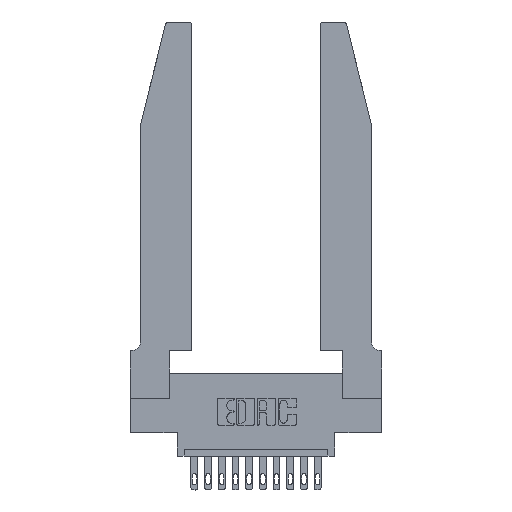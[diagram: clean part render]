
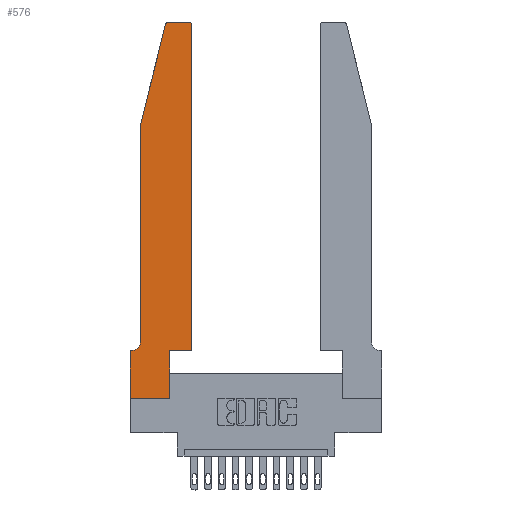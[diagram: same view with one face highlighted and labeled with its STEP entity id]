
A CAD part, top view. The second image highlights one B-rep face of the part: STEP entity #576.
In plain terms, the highlighted planar face has unit normal (0, 0, 1).
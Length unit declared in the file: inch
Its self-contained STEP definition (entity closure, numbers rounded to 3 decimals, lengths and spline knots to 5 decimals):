
#24 = AXIS2_PLACEMENT_3D ( 'NONE', #2159, #11197, #3484 ) ;
#181 = VERTEX_POINT ( 'NONE', #411 ) ;
#197 = EDGE_CURVE ( 'NONE', #6918, #6442, #14031, .T. ) ;
#199 = ORIENTED_EDGE ( 'NONE', *, *, #11106, .T. ) ;
#387 = ORIENTED_EDGE ( 'NONE', *, *, #3849, .T. ) ;
#411 = CARTESIAN_POINT ( 'NONE',  ( 0., 0.35, 0.37 ) ) ;
#432 = EDGE_CURVE ( 'NONE', #5902, #4458, #1122, .T. ) ;
#576 = ADVANCED_FACE ( 'NONE', ( #13816 ), #13175, .T. ) ;
#660 = CARTESIAN_POINT ( 'NONE',  ( 0.2865, 0.35, 0.37 ) ) ;
#712 = DIRECTION ( 'NONE',  ( 0., 1., 0. ) ) ;
#755 = VERTEX_POINT ( 'NONE', #15828 ) ;
#1068 = CARTESIAN_POINT ( 'NONE',  ( 0.0755, 2., 0.37 ) ) ;
#1119 = VECTOR ( 'NONE', #5622, 39.37008 ) ;
#1122 = LINE ( 'NONE', #3855, #8354 ) ;
#1363 = ORIENTED_EDGE ( 'NONE', *, *, #16213, .T. ) ;
#1650 = LINE ( 'NONE', #15632, #12902 ) ;
#1663 = CARTESIAN_POINT ( 'NONE',  ( 0., 0.35, 0.37 ) ) ;
#1938 = CARTESIAN_POINT ( 'NONE',  ( 0.2865, 0.35, 0.37 ) ) ;
#1960 = VERTEX_POINT ( 'NONE', #1938 ) ;
#2159 = CARTESIAN_POINT ( 'NONE',  ( 0.284, 2.72, 0.37 ) ) ;
#2189 = ORIENTED_EDGE ( 'NONE', *, *, #432, .T. ) ;
#2199 = DIRECTION ( 'NONE',  ( -1., 0., 0. ) ) ;
#2227 = EDGE_CURVE ( 'NONE', #9867, #6918, #1650, .T. ) ;
#2305 = DIRECTION ( 'NONE',  ( 0., 0., 1. ) ) ;
#2346 = CARTESIAN_POINT ( 'NONE',  ( 0.4505, 0.35, 0.37 ) ) ;
#2567 = DIRECTION ( 'NONE',  ( 1., 0., 0. ) ) ;
#2919 = LINE ( 'NONE', #660, #11166 ) ;
#3185 = VECTOR ( 'NONE', #3935, 39.37008 ) ;
#3206 = CARTESIAN_POINT ( 'NONE',  ( 0.4505, 0.35, 0.37 ) ) ;
#3394 = CARTESIAN_POINT ( 'NONE',  ( 0.4505, 2.72, 0.37 ) ) ;
#3469 = AXIS2_PLACEMENT_3D ( 'NONE', #1663, #6522, #10651 ) ;
#3484 = DIRECTION ( 'NONE',  ( 1., 0., 0. ) ) ;
#3849 = EDGE_CURVE ( 'NONE', #7775, #12339, #6595, .T. ) ;
#3855 = CARTESIAN_POINT ( 'NONE',  ( 0., 0., 0.37 ) ) ;
#3935 = DIRECTION ( 'NONE',  ( -1., 0., 0. ) ) ;
#4148 = VECTOR ( 'NONE', #11478, 39.37008 ) ;
#4410 = CARTESIAN_POINT ( 'NONE',  ( 0.2865, 0., 0.37 ) ) ;
#4458 = VERTEX_POINT ( 'NONE', #4410 ) ;
#4711 = EDGE_CURVE ( 'NONE', #755, #9867, #16238, .T. ) ;
#4794 = CIRCLE ( 'NONE', #8768, 0.03 ) ;
#4826 = DIRECTION ( 'NONE',  ( -0.239, -0.971, 0. ) ) ;
#4828 = DIRECTION ( 'NONE',  ( 0., -1., 0. ) ) ;
#4886 = ORIENTED_EDGE ( 'NONE', *, *, #6604, .T. ) ;
#5110 = CARTESIAN_POINT ( 'NONE',  ( 0.4505, 0.35, 0.37 ) ) ;
#5537 = LINE ( 'NONE', #5110, #12986 ) ;
#5622 = DIRECTION ( 'NONE',  ( 0., 1., 0. ) ) ;
#5643 = CARTESIAN_POINT ( 'NONE',  ( 0.4205, 2.72, 0.37 ) ) ;
#5808 = DIRECTION ( 'NONE',  ( 0., 0., -1. ) ) ;
#5902 = VERTEX_POINT ( 'NONE', #12167 ) ;
#6265 = CARTESIAN_POINT ( 'NONE',  ( 0.0755, 0.35, 0.37 ) ) ;
#6442 = VERTEX_POINT ( 'NONE', #16561 ) ;
#6520 = LINE ( 'NONE', #6265, #4148 ) ;
#6522 = DIRECTION ( 'NONE',  ( 0., 0., 1. ) ) ;
#6595 = LINE ( 'NONE', #13024, #3185 ) ;
#6604 = EDGE_CURVE ( 'NONE', #6442, #181, #6520, .T. ) ;
#6733 = ORIENTED_EDGE ( 'NONE', *, *, #4711, .T. ) ;
#6918 = VERTEX_POINT ( 'NONE', #12335 ) ;
#6947 = VERTEX_POINT ( 'NONE', #3394 ) ;
#7775 = VERTEX_POINT ( 'NONE', #10259 ) ;
#8217 = EDGE_CURVE ( 'NONE', #12339, #755, #12308, .T. ) ;
#8354 = VECTOR ( 'NONE', #2567, 39.37008 ) ;
#8768 = AXIS2_PLACEMENT_3D ( 'NONE', #5643, #2305, #14742 ) ;
#8792 = ORIENTED_EDGE ( 'NONE', *, *, #8217, .T. ) ;
#9246 = LINE ( 'NONE', #13680, #11465 ) ;
#9390 = VECTOR ( 'NONE', #4826, 39.37008 ) ;
#9867 = VERTEX_POINT ( 'NONE', #15915 ) ;
#10258 = VERTEX_POINT ( 'NONE', #2346 ) ;
#10259 = CARTESIAN_POINT ( 'NONE',  ( 0.4205, 2.75, 0.37 ) ) ;
#10651 = DIRECTION ( 'NONE',  ( 1., 0., 0. ) ) ;
#10722 = ORIENTED_EDGE ( 'NONE', *, *, #197, .T. ) ;
#10838 = EDGE_CURVE ( 'NONE', #181, #5902, #9246, .T. ) ;
#11106 = EDGE_CURVE ( 'NONE', #6947, #7775, #4794, .T. ) ;
#11166 = VECTOR ( 'NONE', #712, 39.37008 ) ;
#11197 = DIRECTION ( 'NONE',  ( 0., 0., 1. ) ) ;
#11465 = VECTOR ( 'NONE', #4828, 39.37008 ) ;
#11478 = DIRECTION ( 'NONE',  ( -1., 0., 0. ) ) ;
#11592 = DIRECTION ( 'NONE',  ( 1., 0., 0. ) ) ;
#11685 = ORIENTED_EDGE ( 'NONE', *, *, #2227, .T. ) ;
#12167 = CARTESIAN_POINT ( 'NONE',  ( 0., 0., 0.37 ) ) ;
#12253 = CARTESIAN_POINT ( 'NONE',  ( 0.0055, 0.42, 0.37 ) ) ;
#12308 = CIRCLE ( 'NONE', #24, 0.03 ) ;
#12335 = CARTESIAN_POINT ( 'NONE',  ( 0.0755, 0.42, 0.37 ) ) ;
#12339 = VERTEX_POINT ( 'NONE', #13051 ) ;
#12366 = LINE ( 'NONE', #3206, #1119 ) ;
#12902 = VECTOR ( 'NONE', #14282, 39.37008 ) ;
#12986 = VECTOR ( 'NONE', #11592, 39.37008 ) ;
#13024 = CARTESIAN_POINT ( 'NONE',  ( 0.2605, 2.75, 0.37 ) ) ;
#13051 = CARTESIAN_POINT ( 'NONE',  ( 0.284, 2.75, 0.37 ) ) ;
#13175 = PLANE ( 'NONE',  #3469 ) ;
#13225 = EDGE_CURVE ( 'NONE', #10258, #6947, #12366, .T. ) ;
#13680 = CARTESIAN_POINT ( 'NONE',  ( 0., 0., 0.37 ) ) ;
#13816 = FACE_OUTER_BOUND ( 'NONE', #14943, .T. ) ;
#14031 = CIRCLE ( 'NONE', #14715, 0.07 ) ;
#14079 = ORIENTED_EDGE ( 'NONE', *, *, #10838, .T. ) ;
#14282 = DIRECTION ( 'NONE',  ( 0., -1., 0. ) ) ;
#14715 = AXIS2_PLACEMENT_3D ( 'NONE', #12253, #5808, #2199 ) ;
#14742 = DIRECTION ( 'NONE',  ( 1., 0., 0. ) ) ;
#14943 = EDGE_LOOP ( 'NONE', ( #387, #8792, #6733, #11685, #10722, #4886, #14079, #2189, #15206, #1363, #15952, #199 ) ) ;
#15206 = ORIENTED_EDGE ( 'NONE', *, *, #16569, .T. ) ;
#15632 = CARTESIAN_POINT ( 'NONE',  ( 0.0755, 2., 0.37 ) ) ;
#15828 = CARTESIAN_POINT ( 'NONE',  ( 0.25487, 2.72718, 0.37 ) ) ;
#15915 = CARTESIAN_POINT ( 'NONE',  ( 0.0755, 2., 0.37 ) ) ;
#15952 = ORIENTED_EDGE ( 'NONE', *, *, #13225, .T. ) ;
#16213 = EDGE_CURVE ( 'NONE', #1960, #10258, #5537, .T. ) ;
#16238 = LINE ( 'NONE', #1068, #9390 ) ;
#16561 = CARTESIAN_POINT ( 'NONE',  ( 0.0055, 0.35, 0.37 ) ) ;
#16569 = EDGE_CURVE ( 'NONE', #4458, #1960, #2919, .T. ) ;
